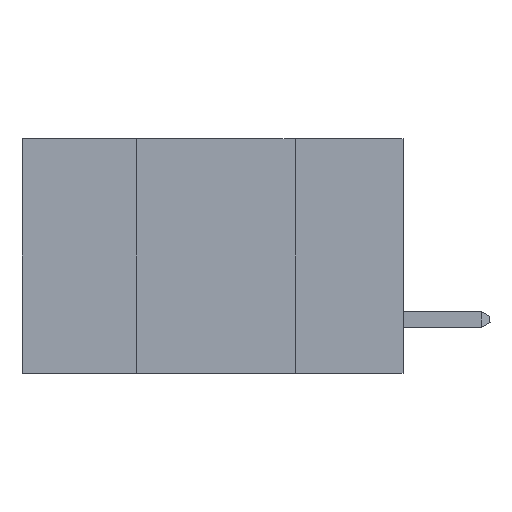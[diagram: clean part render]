
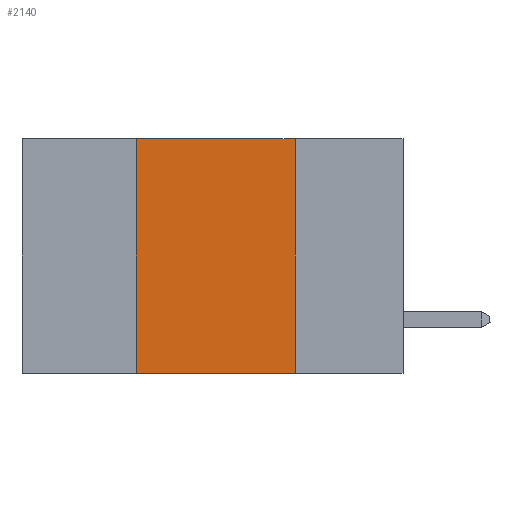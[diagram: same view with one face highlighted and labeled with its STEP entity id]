
A CAD part, left-side view. The second image highlights one B-rep face of the part: STEP entity #2140.
In plain terms, the highlighted planar face has unit normal (-1, 0, 0).
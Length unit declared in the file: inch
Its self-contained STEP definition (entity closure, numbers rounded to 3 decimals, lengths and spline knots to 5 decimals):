
#85 = VECTOR ( 'NONE', #16478, 39.37008 ) ;
#344 = CARTESIAN_POINT ( 'NONE',  ( 0., 0.42, 0. ) ) ;
#937 = VERTEX_POINT ( 'NONE', #15108 ) ;
#1136 = CARTESIAN_POINT ( 'NONE',  ( 0., 0.6, 0. ) ) ;
#1398 = EDGE_CURVE ( 'NONE', #10725, #8932, #5476, .T. ) ;
#1567 = VECTOR ( 'NONE', #19849, 39.37008 ) ;
#2140 = ADVANCED_FACE ( 'NONE', ( #8781 ), #7560, .F. ) ;
#3939 = ORIENTED_EDGE ( 'NONE', *, *, #6048, .F. ) ;
#4303 = CARTESIAN_POINT ( 'NONE',  ( 0., 0.17, 0. ) ) ;
#5000 = CARTESIAN_POINT ( 'NONE',  ( 0., 0.17, -0.37 ) ) ;
#5476 = LINE ( 'NONE', #9829, #85 ) ;
#5923 = CARTESIAN_POINT ( 'NONE',  ( 0., 0.42, 0. ) ) ;
#6048 = EDGE_CURVE ( 'NONE', #937, #7133, #18782, .T. ) ;
#7133 = VERTEX_POINT ( 'NONE', #5923 ) ;
#7560 = PLANE ( 'NONE',  #16882 ) ;
#8675 = LINE ( 'NONE', #17341, #18156 ) ;
#8781 = FACE_OUTER_BOUND ( 'NONE', #15933, .T. ) ;
#8932 = VERTEX_POINT ( 'NONE', #5000 ) ;
#9188 = DIRECTION ( 'NONE',  ( 1., 0., 0. ) ) ;
#9829 = CARTESIAN_POINT ( 'NONE',  ( 0., 0.17, 0. ) ) ;
#10725 = VERTEX_POINT ( 'NONE', #4303 ) ;
#12335 = DIRECTION ( 'NONE',  ( 0., -1., 0. ) ) ;
#13271 = VECTOR ( 'NONE', #13532, 39.37008 ) ;
#13532 = DIRECTION ( 'NONE',  ( 0., -1., 0. ) ) ;
#14306 = ORIENTED_EDGE ( 'NONE', *, *, #15596, .T. ) ;
#15108 = CARTESIAN_POINT ( 'NONE',  ( 0., 0.42, -0.37 ) ) ;
#15481 = CARTESIAN_POINT ( 'NONE',  ( 0., 0.6, -0.37 ) ) ;
#15596 = EDGE_CURVE ( 'NONE', #937, #8932, #21260, .T. ) ;
#15843 = DIRECTION ( 'NONE',  ( 0., 0., -1. ) ) ;
#15933 = EDGE_LOOP ( 'NONE', ( #16731, #16680, #3939, #14306 ) ) ;
#16478 = DIRECTION ( 'NONE',  ( 0., 0., -1. ) ) ;
#16680 = ORIENTED_EDGE ( 'NONE', *, *, #17337, .F. ) ;
#16731 = ORIENTED_EDGE ( 'NONE', *, *, #1398, .F. ) ;
#16882 = AXIS2_PLACEMENT_3D ( 'NONE', #1136, #9188, #15843 ) ;
#17337 = EDGE_CURVE ( 'NONE', #7133, #10725, #8675, .T. ) ;
#17341 = CARTESIAN_POINT ( 'NONE',  ( 0., 0.6, 0. ) ) ;
#18156 = VECTOR ( 'NONE', #12335, 39.37008 ) ;
#18782 = LINE ( 'NONE', #344, #1567 ) ;
#19849 = DIRECTION ( 'NONE',  ( 0., 0., 1. ) ) ;
#21260 = LINE ( 'NONE', #15481, #13271 ) ;
